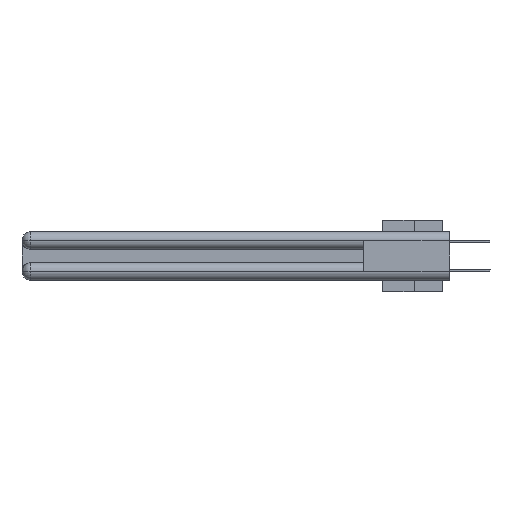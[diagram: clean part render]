
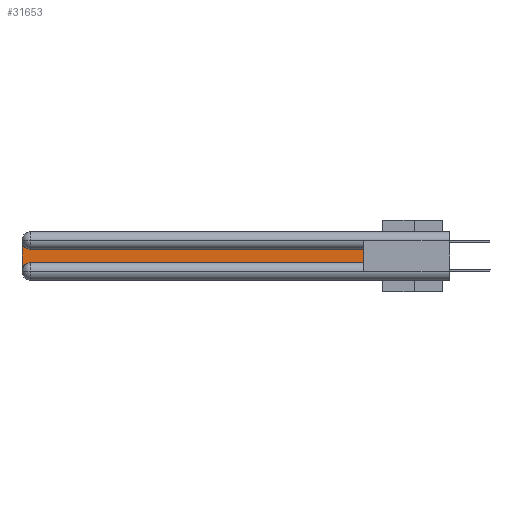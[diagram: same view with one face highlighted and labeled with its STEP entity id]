
A CAD part, left-side view. The second image highlights one B-rep face of the part: STEP entity #31653.
In plain terms, the highlighted planar face has unit normal (-1, 0, 0).
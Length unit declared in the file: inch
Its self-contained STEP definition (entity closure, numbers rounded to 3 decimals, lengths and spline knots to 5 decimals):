
#1224 = CIRCLE ( 'NONE', #5897, 0.06 ) ;
#1308 = AXIS2_PLACEMENT_3D ( 'NONE', #7941, #26043, #15529 ) ;
#1321 = ORIENTED_EDGE ( 'NONE', *, *, #7140, .T. ) ;
#1654 = VERTEX_POINT ( 'NONE', #17700 ) ;
#1808 = DIRECTION ( 'NONE',  ( 0., 0., -1. ) ) ;
#1941 = CARTESIAN_POINT ( 'NONE',  ( 0.075, 3., -0.2775 ) ) ;
#2657 = CARTESIAN_POINT ( 'NONE',  ( 0.075, 0.6, -0.2175 ) ) ;
#2711 = VERTEX_POINT ( 'NONE', #7344 ) ;
#3602 = LINE ( 'NONE', #2657, #24473 ) ;
#4678 = DIRECTION ( 'NONE',  ( 1., 0., 0. ) ) ;
#5343 = PLANE ( 'NONE',  #1308 ) ;
#5368 = LINE ( 'NONE', #9664, #25807 ) ;
#5897 = AXIS2_PLACEMENT_3D ( 'NONE', #27867, #4678, #6855 ) ;
#5900 = FACE_OUTER_BOUND ( 'NONE', #27019, .T. ) ;
#6315 = VERTEX_POINT ( 'NONE', #24099 ) ;
#6855 = DIRECTION ( 'NONE',  ( 0., 0., -1. ) ) ;
#7140 = EDGE_CURVE ( 'NONE', #22806, #2711, #24635, .T. ) ;
#7215 = DIRECTION ( 'NONE',  ( 0., 1., 0. ) ) ;
#7307 = CARTESIAN_POINT ( 'NONE',  ( 0.075, 3., -0.0625 ) ) ;
#7344 = CARTESIAN_POINT ( 'NONE',  ( 0.075, 0.6, -0.1225 ) ) ;
#7941 = CARTESIAN_POINT ( 'NONE',  ( 0.075, 3., -0.1225 ) ) ;
#8988 = EDGE_CURVE ( 'NONE', #1654, #22806, #3602, .T. ) ;
#9636 = ORIENTED_EDGE ( 'NONE', *, *, #24924, .T. ) ;
#9664 = CARTESIAN_POINT ( 'NONE',  ( 0.075, 3., -0.2175 ) ) ;
#10931 = CARTESIAN_POINT ( 'NONE',  ( 0.075, 0.6, -0.2175 ) ) ;
#11583 = VERTEX_POINT ( 'NONE', #7307 ) ;
#11971 = EDGE_CURVE ( 'NONE', #29107, #1654, #14516, .T. ) ;
#12776 = VECTOR ( 'NONE', #21772, 39.37008 ) ;
#14363 = DIRECTION ( 'NONE',  ( 1., 0., 0. ) ) ;
#14516 = CIRCLE ( 'NONE', #33073, 0.06 ) ;
#15529 = DIRECTION ( 'NONE',  ( 0., 0., -1. ) ) ;
#16626 = CARTESIAN_POINT ( 'NONE',  ( 0.075, 0.6, -0.2175 ) ) ;
#17690 = CARTESIAN_POINT ( 'NONE',  ( 0.075, 2.94, -0.2775 ) ) ;
#17700 = CARTESIAN_POINT ( 'NONE',  ( 0.075, 2.94, -0.2175 ) ) ;
#20470 = EDGE_CURVE ( 'NONE', #6315, #11583, #1224, .T. ) ;
#21065 = EDGE_CURVE ( 'NONE', #11583, #29107, #5368, .T. ) ;
#21772 = DIRECTION ( 'NONE',  ( 0., 0., 1. ) ) ;
#21881 = VECTOR ( 'NONE', #7215, 39.37008 ) ;
#22806 = VERTEX_POINT ( 'NONE', #10931 ) ;
#24099 = CARTESIAN_POINT ( 'NONE',  ( 0.075, 2.94, -0.1225 ) ) ;
#24473 = VECTOR ( 'NONE', #33767, 39.37008 ) ;
#24635 = LINE ( 'NONE', #16626, #12776 ) ;
#24924 = EDGE_CURVE ( 'NONE', #2711, #6315, #28848, .T. ) ;
#25807 = VECTOR ( 'NONE', #1808, 39.37008 ) ;
#26043 = DIRECTION ( 'NONE',  ( 1., 0., 0. ) ) ;
#27019 = EDGE_LOOP ( 'NONE', ( #9636, #32111, #31780, #31527, #33518, #1321 ) ) ;
#27461 = CARTESIAN_POINT ( 'NONE',  ( 0.075, 0.6, -0.1225 ) ) ;
#27867 = CARTESIAN_POINT ( 'NONE',  ( 0.075, 2.94, -0.0625 ) ) ;
#28053 = DIRECTION ( 'NONE',  ( 0., 0., -1. ) ) ;
#28848 = LINE ( 'NONE', #27461, #21881 ) ;
#29107 = VERTEX_POINT ( 'NONE', #1941 ) ;
#31527 = ORIENTED_EDGE ( 'NONE', *, *, #11971, .T. ) ;
#31653 = ADVANCED_FACE ( 'NONE', ( #5900 ), #5343, .F. ) ;
#31780 = ORIENTED_EDGE ( 'NONE', *, *, #21065, .T. ) ;
#32111 = ORIENTED_EDGE ( 'NONE', *, *, #20470, .T. ) ;
#33073 = AXIS2_PLACEMENT_3D ( 'NONE', #17690, #14363, #28053 ) ;
#33518 = ORIENTED_EDGE ( 'NONE', *, *, #8988, .T. ) ;
#33767 = DIRECTION ( 'NONE',  ( 0., -1., 0. ) ) ;
